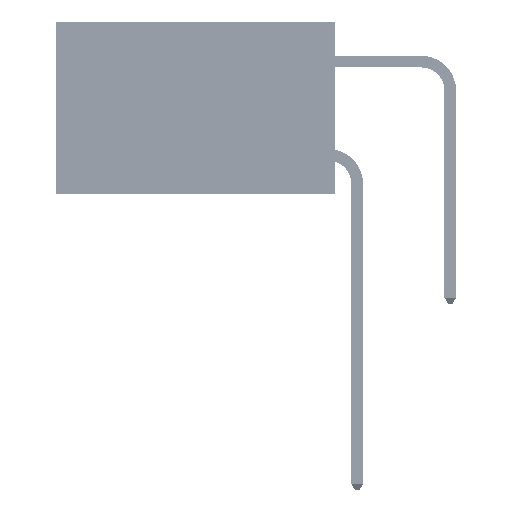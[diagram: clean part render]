
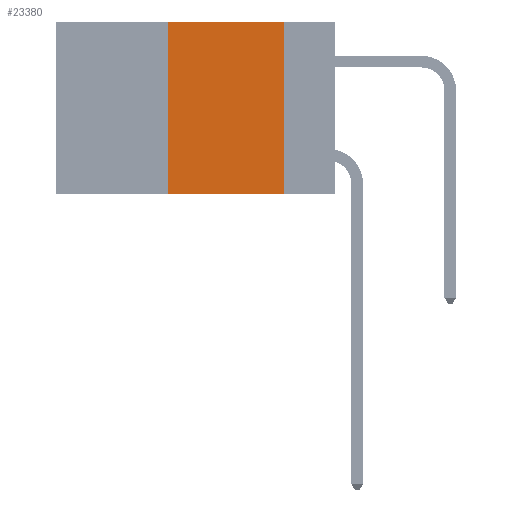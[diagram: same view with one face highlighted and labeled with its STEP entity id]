
A CAD part, left-side view. The second image highlights one B-rep face of the part: STEP entity #23380.
In plain terms, the highlighted planar face has unit normal (-1, 0, 0).
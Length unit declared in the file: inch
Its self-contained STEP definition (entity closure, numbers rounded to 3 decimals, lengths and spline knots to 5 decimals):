
#3217 = LINE ( 'NONE', #14373, #22924 ) ;
#5333 = AXIS2_PLACEMENT_3D ( 'NONE', #25248, #5966, #14374 ) ;
#5966 = DIRECTION ( 'NONE',  ( 1., 0., 0. ) ) ;
#6672 = ORIENTED_EDGE ( 'NONE', *, *, #33072, .F. ) ;
#7474 = ORIENTED_EDGE ( 'NONE', *, *, #27871, .F. ) ;
#7849 = VERTEX_POINT ( 'NONE', #46930 ) ;
#7937 = DIRECTION ( 'NONE',  ( 0., -1., 0. ) ) ;
#10306 = CARTESIAN_POINT ( 'NONE',  ( 0., 0.6, -0.37 ) ) ;
#11860 = CARTESIAN_POINT ( 'NONE',  ( 0., 0.11, 0. ) ) ;
#14261 = DIRECTION ( 'NONE',  ( 0., -1., 0. ) ) ;
#14373 = CARTESIAN_POINT ( 'NONE',  ( 0., 0.36, 0. ) ) ;
#14374 = DIRECTION ( 'NONE',  ( 0., 0., -1. ) ) ;
#15121 = LINE ( 'NONE', #18330, #28354 ) ;
#17600 = VECTOR ( 'NONE', #14261, 39.37008 ) ;
#18330 = CARTESIAN_POINT ( 'NONE',  ( 0., 0.6, 0. ) ) ;
#18848 = CARTESIAN_POINT ( 'NONE',  ( 0., 0.36, 0. ) ) ;
#20049 = EDGE_LOOP ( 'NONE', ( #32047, #6672, #7474, #47863 ) ) ;
#20649 = EDGE_CURVE ( 'NONE', #47804, #44067, #33057, .T. ) ;
#21792 = DIRECTION ( 'NONE',  ( 0., 0., 1. ) ) ;
#22924 = VECTOR ( 'NONE', #21792, 39.37008 ) ;
#23234 = LINE ( 'NONE', #11860, #23869 ) ;
#23380 = ADVANCED_FACE ( 'NONE', ( #32175 ), #39849, .F. ) ;
#23869 = VECTOR ( 'NONE', #26953, 39.37008 ) ;
#25248 = CARTESIAN_POINT ( 'NONE',  ( 0., 0.6, 0. ) ) ;
#26953 = DIRECTION ( 'NONE',  ( 0., 0., -1. ) ) ;
#27861 = CARTESIAN_POINT ( 'NONE',  ( 0., 0.11, -0.37 ) ) ;
#27871 = EDGE_CURVE ( 'NONE', #47804, #33879, #3217, .T. ) ;
#28354 = VECTOR ( 'NONE', #7937, 39.37008 ) ;
#32047 = ORIENTED_EDGE ( 'NONE', *, *, #48468, .F. ) ;
#32175 = FACE_OUTER_BOUND ( 'NONE', #20049, .T. ) ;
#33057 = LINE ( 'NONE', #10306, #17600 ) ;
#33072 = EDGE_CURVE ( 'NONE', #33879, #7849, #15121, .T. ) ;
#33879 = VERTEX_POINT ( 'NONE', #18848 ) ;
#36919 = CARTESIAN_POINT ( 'NONE',  ( 0., 0.36, -0.37 ) ) ;
#39849 = PLANE ( 'NONE',  #5333 ) ;
#44067 = VERTEX_POINT ( 'NONE', #27861 ) ;
#46930 = CARTESIAN_POINT ( 'NONE',  ( 0., 0.11, 0. ) ) ;
#47804 = VERTEX_POINT ( 'NONE', #36919 ) ;
#47863 = ORIENTED_EDGE ( 'NONE', *, *, #20649, .T. ) ;
#48468 = EDGE_CURVE ( 'NONE', #7849, #44067, #23234, .T. ) ;
